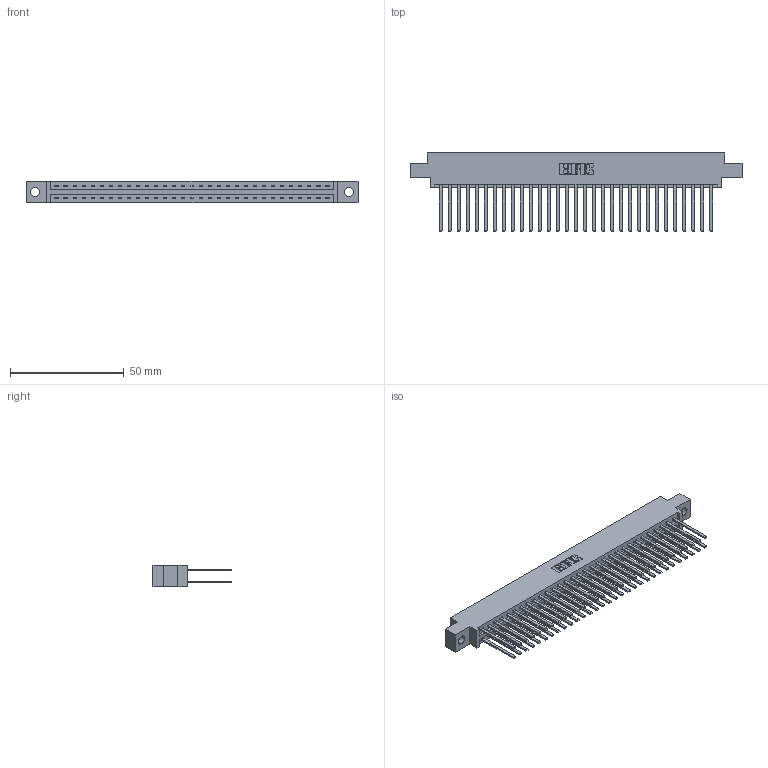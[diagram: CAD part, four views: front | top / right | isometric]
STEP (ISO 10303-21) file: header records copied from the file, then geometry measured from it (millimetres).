
FILE_DESCRIPTION (( 'STEP AP203' ), '1' );
FILE_NAME ('337-062-544-804.STEP', '2018-08-11T04:29:48', ( '' ), ( '' ), 'SwSTEP 2.0', 'SolidWorks 2016', '' );
FILE_SCHEMA (( 'CONFIG_CONTROL_DESIGN' ));
Length unit declared in the file: inch
Products named in the file (3): 337 Part_0.170 Offset - 0.156 Dia-TH; 345-292-001_345-293-144; 337-062-544-804
Assembly tree (63 placements, depth 2):
  337-062-544-804
    337 Part_0.170 Offset - 0.156 Dia-TH
    345-292-001_345-293-144  x62
Bounding box: 145.85 x 34.3 x 9.4 mm (x, y, z)
Volume: 15887.8 mm3; surface area: 20598.8 mm2
Topology: 63 solids, 63 shells, 3094 faces, 9189 edges, 6042 vertices
Faces by surface type: plane 2182, cylinder 912
Entity records: 25409 total; most frequent: CARTESIAN_POINT 4290, ORIENTED_EDGE 4226, DIRECTION 3665, EDGE_CURVE 2113, LINE 1989, VECTOR 1989, VERTEX_POINT 1406, AXIS2_PLACEMENT_3D 838
